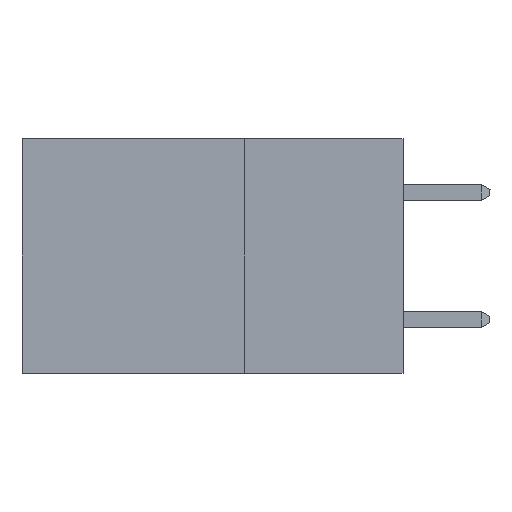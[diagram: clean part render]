
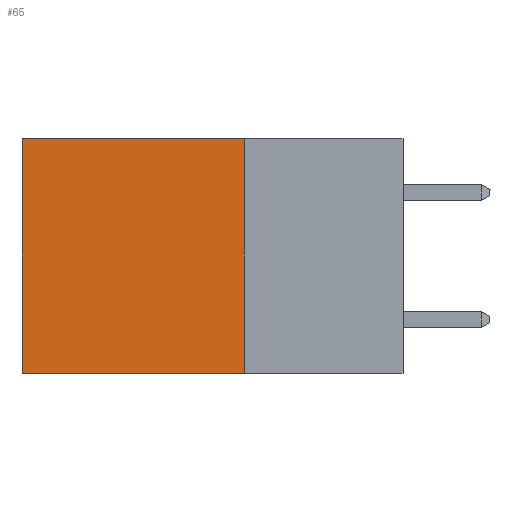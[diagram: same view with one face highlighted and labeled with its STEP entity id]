
A CAD part, left-side view. The second image highlights one B-rep face of the part: STEP entity #65.
In plain terms, the highlighted planar face has unit normal (-1, 0, 0).
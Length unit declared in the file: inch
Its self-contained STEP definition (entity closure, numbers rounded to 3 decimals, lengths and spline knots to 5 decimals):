
#65 = ADVANCED_FACE ( 'NONE', ( #24351 ), #24126, .F. ) ;
#875 = DIRECTION ( 'NONE',  ( 0., 0., -1. ) ) ;
#1810 = VERTEX_POINT ( 'NONE', #4892 ) ;
#3633 = VECTOR ( 'NONE', #4532, 39.37008 ) ;
#4532 = DIRECTION ( 'NONE',  ( 0., 0., -1. ) ) ;
#4892 = CARTESIAN_POINT ( 'NONE',  ( 0.2875, 0.25, 0. ) ) ;
#5389 = VERTEX_POINT ( 'NONE', #14223 ) ;
#5401 = CARTESIAN_POINT ( 'NONE',  ( 0.2875, 0.25, 0. ) ) ;
#7939 = CARTESIAN_POINT ( 'NONE',  ( 0.2875, 0.6, 0. ) ) ;
#8582 = DIRECTION ( 'NONE',  ( 0., 1., 0. ) ) ;
#9798 = ORIENTED_EDGE ( 'NONE', *, *, #27263, .T. ) ;
#9889 = LINE ( 'NONE', #20817, #3633 ) ;
#10111 = DIRECTION ( 'NONE',  ( 1., 0., 0. ) ) ;
#10723 = DIRECTION ( 'NONE',  ( 0., 1., 0. ) ) ;
#11462 = AXIS2_PLACEMENT_3D ( 'NONE', #5401, #10111, #26455 ) ;
#12027 = CARTESIAN_POINT ( 'NONE',  ( 0.2875, 0.25, -0.37 ) ) ;
#13663 = VECTOR ( 'NONE', #10723, 39.37008 ) ;
#14223 = CARTESIAN_POINT ( 'NONE',  ( 0.2875, 0.6, 0. ) ) ;
#14728 = ORIENTED_EDGE ( 'NONE', *, *, #28837, .F. ) ;
#15422 = VECTOR ( 'NONE', #8582, 39.37008 ) ;
#17138 = EDGE_CURVE ( 'NONE', #1810, #5389, #26806, .T. ) ;
#17380 = LINE ( 'NONE', #7939, #28318 ) ;
#17676 = ORIENTED_EDGE ( 'NONE', *, *, #19812, .F. ) ;
#19812 = EDGE_CURVE ( 'NONE', #1810, #23078, #9889, .T. ) ;
#20049 = CARTESIAN_POINT ( 'NONE',  ( 0.2875, 0.25, 0. ) ) ;
#20248 = CARTESIAN_POINT ( 'NONE',  ( 0.2875, 0.25, -0.37 ) ) ;
#20817 = CARTESIAN_POINT ( 'NONE',  ( 0.2875, 0.25, 0. ) ) ;
#22835 = CARTESIAN_POINT ( 'NONE',  ( 0.2875, 0.6, -0.37 ) ) ;
#23078 = VERTEX_POINT ( 'NONE', #12027 ) ;
#24126 = PLANE ( 'NONE',  #11462 ) ;
#24351 = FACE_OUTER_BOUND ( 'NONE', #28064, .T. ) ;
#26455 = DIRECTION ( 'NONE',  ( 0., 0., -1. ) ) ;
#26806 = LINE ( 'NONE', #20049, #13663 ) ;
#26971 = ORIENTED_EDGE ( 'NONE', *, *, #17138, .T. ) ;
#27115 = LINE ( 'NONE', #20248, #15422 ) ;
#27263 = EDGE_CURVE ( 'NONE', #5389, #27507, #17380, .T. ) ;
#27507 = VERTEX_POINT ( 'NONE', #22835 ) ;
#28064 = EDGE_LOOP ( 'NONE', ( #9798, #14728, #17676, #26971 ) ) ;
#28318 = VECTOR ( 'NONE', #875, 39.37008 ) ;
#28837 = EDGE_CURVE ( 'NONE', #23078, #27507, #27115, .T. ) ;
